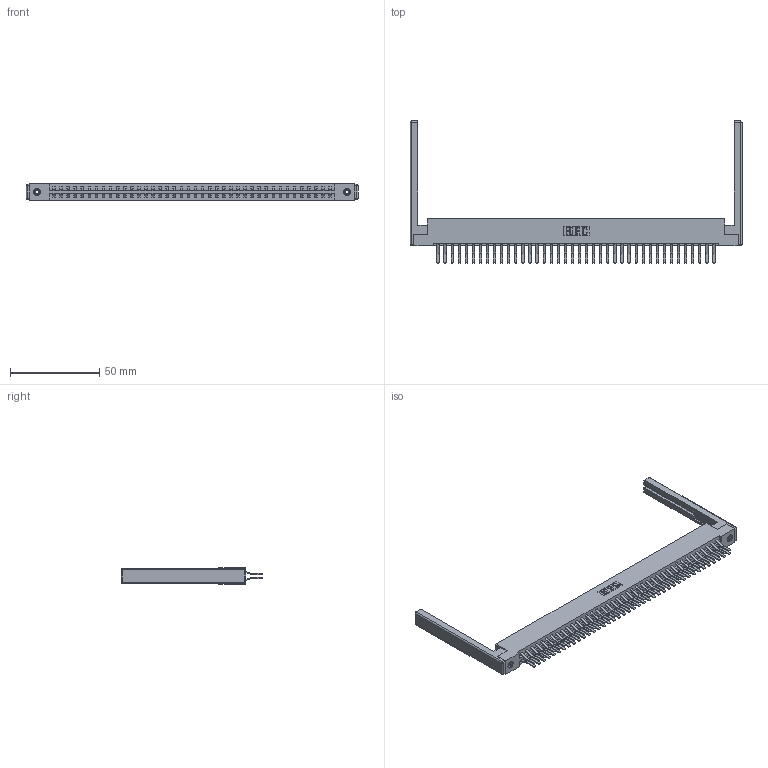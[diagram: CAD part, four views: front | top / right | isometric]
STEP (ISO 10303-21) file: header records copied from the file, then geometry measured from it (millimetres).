
FILE_DESCRIPTION (( 'STEP AP203' ), '1' );
FILE_NAME ('337-080-560-268.STEP', '2019-10-10T12:41:07', ( '' ), ( '' ), 'SwSTEP 2.0', 'SolidWorks 2016', '' );
FILE_SCHEMA (( 'CONFIG_CONTROL_DESIGN' ));
Length unit declared in the file: inch
Products named in the file (5): 345-250-001_345-250-001-102; 337-080-560-268; 307-220-068; 337 Part_Flush Mounting Lugs - 0.156 Dia-TI; 345-292-001_560 Tail
Assembly tree (85 placements, depth 2):
  337-080-560-268
    337 Part_Flush Mounting Lugs - 0.156 Dia-TI
    345-292-001_560 Tail  x80
    345-250-001_345-250-001-102  x2
    307-220-068  x2
Bounding box: 185.93 x 79.52 x 9.4 mm (x, y, z)
Volume: 24477.1 mm3; surface area: 28247 mm2
Topology: 85 solids, 85 shells, 4748 faces, 14061 edges, 9246 vertices
Faces by surface type: plane 3198, cylinder 1526, cone 12, sphere 8, torus 4
Entity records: 34120 total; most frequent: CARTESIAN_POINT 5715, ORIENTED_EDGE 5640, DIRECTION 4938, EDGE_CURVE 2820, LINE 2638, VECTOR 2638, VERTEX_POINT 1870, AXIS2_PLACEMENT_3D 1150
